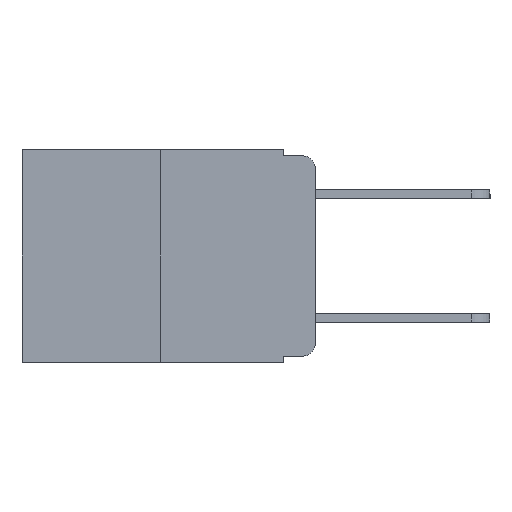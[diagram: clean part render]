
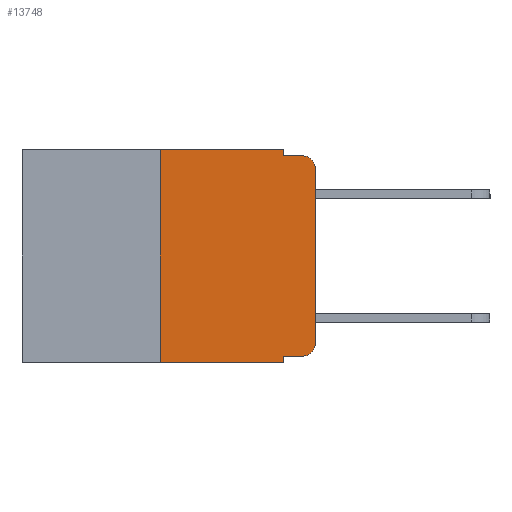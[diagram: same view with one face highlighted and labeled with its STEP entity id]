
A CAD part, left-side view. The second image highlights one B-rep face of the part: STEP entity #13748.
In plain terms, the highlighted planar face has unit normal (-1, 0, 0).
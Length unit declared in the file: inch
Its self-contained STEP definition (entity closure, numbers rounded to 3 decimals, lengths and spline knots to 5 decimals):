
#56 = ORIENTED_EDGE ( 'NONE', *, *, #12286, .F. ) ;
#360 = ORIENTED_EDGE ( 'NONE', *, *, #16629, .F. ) ;
#1198 = CARTESIAN_POINT ( 'NONE',  ( 0., 0.25, 0. ) ) ;
#1294 = CARTESIAN_POINT ( 'NONE',  ( 0., 0.02, -0.03 ) ) ;
#1298 = DIRECTION ( 'NONE',  ( 0., -1., 0. ) ) ;
#1430 = DIRECTION ( 'NONE',  ( 0., -1., 0. ) ) ;
#2065 = ORIENTED_EDGE ( 'NONE', *, *, #16534, .F. ) ;
#2532 = VERTEX_POINT ( 'NONE', #16233 ) ;
#2825 = VECTOR ( 'NONE', #12016, 39.37008 ) ;
#3087 = DIRECTION ( 'NONE',  ( 0., 0., -1. ) ) ;
#3165 = VERTEX_POINT ( 'NONE', #5985 ) ;
#3225 = CARTESIAN_POINT ( 'NONE',  ( 0., 0.051, 0. ) ) ;
#3239 = DIRECTION ( 'NONE',  ( 0., 0., 1. ) ) ;
#3537 = ORIENTED_EDGE ( 'NONE', *, *, #16342, .T. ) ;
#3694 = ORIENTED_EDGE ( 'NONE', *, *, #16532, .F. ) ;
#3724 = LINE ( 'NONE', #17896, #17230 ) ;
#3973 = ORIENTED_EDGE ( 'NONE', *, *, #16367, .T. ) ;
#4103 = PLANE ( 'NONE',  #10302 ) ;
#4808 = DIRECTION ( 'NONE',  ( 0., -1., 0. ) ) ;
#4919 = LINE ( 'NONE', #14430, #11646 ) ;
#4952 = CARTESIAN_POINT ( 'NONE',  ( 0., 0.473, -0.343 ) ) ;
#5622 = VERTEX_POINT ( 'NONE', #15366 ) ;
#5957 = CIRCLE ( 'NONE', #10783, 0.02 ) ;
#5985 = CARTESIAN_POINT ( 'NONE',  ( 0., 0.02, -0.01 ) ) ;
#6013 = CIRCLE ( 'NONE', #17506, 0.02 ) ;
#6365 = DIRECTION ( 'NONE',  ( 0., 0., 1. ) ) ;
#6611 = CARTESIAN_POINT ( 'NONE',  ( 0., 0.051, 0. ) ) ;
#6902 = VERTEX_POINT ( 'NONE', #8257 ) ;
#6972 = ORIENTED_EDGE ( 'NONE', *, *, #17791, .T. ) ;
#7163 = VECTOR ( 'NONE', #9166, 39.37008 ) ;
#7400 = CARTESIAN_POINT ( 'NONE',  ( 0., 0.051, -0.343 ) ) ;
#7471 = DIRECTION ( 'NONE',  ( -1., 0., 0. ) ) ;
#7770 = VERTEX_POINT ( 'NONE', #9341 ) ;
#7864 = VERTEX_POINT ( 'NONE', #6611 ) ;
#8224 = CARTESIAN_POINT ( 'NONE',  ( 0., 0.02, -0.333 ) ) ;
#8257 = CARTESIAN_POINT ( 'NONE',  ( 0., 0.051, -0.333 ) ) ;
#8502 = LINE ( 'NONE', #4952, #17663 ) ;
#8911 = ORIENTED_EDGE ( 'NONE', *, *, #17772, .T. ) ;
#9012 = ORIENTED_EDGE ( 'NONE', *, *, #17728, .F. ) ;
#9166 = DIRECTION ( 'NONE',  ( 0., 0., -1. ) ) ;
#9341 = CARTESIAN_POINT ( 'NONE',  ( 0., 0.25, 0. ) ) ;
#9452 = FACE_OUTER_BOUND ( 'NONE', #11107, .T. ) ;
#9575 = VERTEX_POINT ( 'NONE', #8224 ) ;
#9817 = VECTOR ( 'NONE', #13971, 39.37008 ) ;
#10239 = LINE ( 'NONE', #17491, #9817 ) ;
#10302 = AXIS2_PLACEMENT_3D ( 'NONE', #11400, #17382, #13906 ) ;
#10538 = CARTESIAN_POINT ( 'NONE',  ( 0., 0.051, 0. ) ) ;
#10783 = AXIS2_PLACEMENT_3D ( 'NONE', #1294, #11917, #3087 ) ;
#10848 = LINE ( 'NONE', #1198, #17698 ) ;
#11107 = EDGE_LOOP ( 'NONE', ( #8911, #11485, #9012, #360, #56, #2065, #6972, #3694, #3537, #3973 ) ) ;
#11400 = CARTESIAN_POINT ( 'NONE',  ( 0., 0.473, 0. ) ) ;
#11485 = ORIENTED_EDGE ( 'NONE', *, *, #17708, .T. ) ;
#11646 = VECTOR ( 'NONE', #3239, 39.37008 ) ;
#11917 = DIRECTION ( 'NONE',  ( -1., 0., 0. ) ) ;
#12016 = DIRECTION ( 'NONE',  ( 0., 0., -1. ) ) ;
#12286 = EDGE_CURVE ( 'NONE', #7770, #7864, #3724, .T. ) ;
#12444 = VECTOR ( 'NONE', #4808, 39.37008 ) ;
#13080 = VERTEX_POINT ( 'NONE', #17937 ) ;
#13748 = ADVANCED_FACE ( 'NONE', ( #9452 ), #4103, .F. ) ;
#13906 = DIRECTION ( 'NONE',  ( 0., 0., -1. ) ) ;
#13971 = DIRECTION ( 'NONE',  ( 0., -1., 0. ) ) ;
#14191 = LINE ( 'NONE', #10538, #7163 ) ;
#14430 = CARTESIAN_POINT ( 'NONE',  ( 0., 0., 0. ) ) ;
#15234 = CARTESIAN_POINT ( 'NONE',  ( 0., 0.02, -0.313 ) ) ;
#15366 = CARTESIAN_POINT ( 'NONE',  ( 0., 0.051, -0.01 ) ) ;
#15630 = LINE ( 'NONE', #17891, #12444 ) ;
#16233 = CARTESIAN_POINT ( 'NONE',  ( 0., 0., -0.313 ) ) ;
#16342 = EDGE_CURVE ( 'NONE', #6902, #9575, #10239, .T. ) ;
#16348 = VERTEX_POINT ( 'NONE', #7400 ) ;
#16367 = EDGE_CURVE ( 'NONE', #9575, #2532, #6013, .T. ) ;
#16442 = DIRECTION ( 'NONE',  ( 0., 0., -1. ) ) ;
#16532 = EDGE_CURVE ( 'NONE', #6902, #16348, #14191, .T. ) ;
#16534 = EDGE_CURVE ( 'NONE', #13080, #7770, #10848, .T. ) ;
#16629 = EDGE_CURVE ( 'NONE', #7864, #5622, #16986, .T. ) ;
#16986 = LINE ( 'NONE', #3225, #2825 ) ;
#17026 = CARTESIAN_POINT ( 'NONE',  ( 0., 0., -0.03 ) ) ;
#17230 = VECTOR ( 'NONE', #1298, 39.37008 ) ;
#17382 = DIRECTION ( 'NONE',  ( 1., 0., 0. ) ) ;
#17452 = VERTEX_POINT ( 'NONE', #17026 ) ;
#17491 = CARTESIAN_POINT ( 'NONE',  ( 0., 0.051, -0.333 ) ) ;
#17506 = AXIS2_PLACEMENT_3D ( 'NONE', #15234, #7471, #16442 ) ;
#17663 = VECTOR ( 'NONE', #1430, 39.37008 ) ;
#17698 = VECTOR ( 'NONE', #6365, 39.37008 ) ;
#17708 = EDGE_CURVE ( 'NONE', #17452, #3165, #5957, .T. ) ;
#17728 = EDGE_CURVE ( 'NONE', #5622, #3165, #15630, .T. ) ;
#17772 = EDGE_CURVE ( 'NONE', #2532, #17452, #4919, .T. ) ;
#17791 = EDGE_CURVE ( 'NONE', #13080, #16348, #8502, .T. ) ;
#17891 = CARTESIAN_POINT ( 'NONE',  ( 0., 0.051, -0.01 ) ) ;
#17896 = CARTESIAN_POINT ( 'NONE',  ( 0., 0.473, 0. ) ) ;
#17937 = CARTESIAN_POINT ( 'NONE',  ( 0., 0.25, -0.343 ) ) ;
